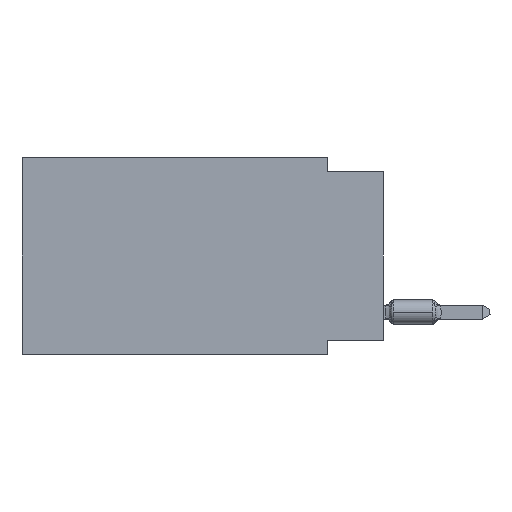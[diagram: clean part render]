
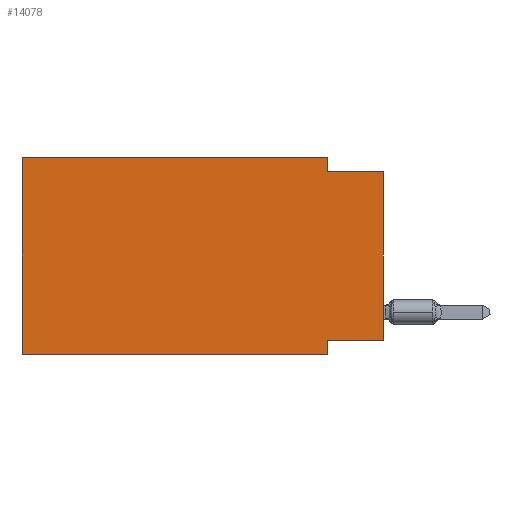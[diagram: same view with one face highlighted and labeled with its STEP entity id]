
A CAD part, left-side view. The second image highlights one B-rep face of the part: STEP entity #14078.
In plain terms, the highlighted planar face has unit normal (-1, 0, 0).
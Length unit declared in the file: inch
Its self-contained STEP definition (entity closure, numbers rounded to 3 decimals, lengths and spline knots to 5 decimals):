
#83 = VERTEX_POINT ( 'NONE', #13696 ) ;
#477 = EDGE_CURVE ( 'NONE', #13368, #14220, #11567, .T. ) ;
#613 = LINE ( 'NONE', #16002, #7493 ) ;
#871 = DIRECTION ( 'NONE',  ( 0., 0., 1. ) ) ;
#1409 = EDGE_CURVE ( 'NONE', #14233, #17961, #1791, .T. ) ;
#1791 = LINE ( 'NONE', #1878, #2820 ) ;
#1878 = CARTESIAN_POINT ( 'NONE',  ( 0., 0., -0.325 ) ) ;
#1926 = CARTESIAN_POINT ( 'NONE',  ( 0., 0.1, -0.025 ) ) ;
#2315 = VECTOR ( 'NONE', #11634, 39.37008 ) ;
#2380 = CARTESIAN_POINT ( 'NONE',  ( 0., 0.645, -0.35 ) ) ;
#2670 = FACE_OUTER_BOUND ( 'NONE', #18024, .T. ) ;
#2742 = ORIENTED_EDGE ( 'NONE', *, *, #7738, .F. ) ;
#2820 = VECTOR ( 'NONE', #7370, 39.37008 ) ;
#2941 = LINE ( 'NONE', #5693, #15136 ) ;
#3067 = VERTEX_POINT ( 'NONE', #17704 ) ;
#3193 = CARTESIAN_POINT ( 'NONE',  ( 0., 0., -0.325 ) ) ;
#3515 = AXIS2_PLACEMENT_3D ( 'NONE', #15423, #4151, #9726 ) ;
#3712 = CARTESIAN_POINT ( 'NONE',  ( 0., 0., -0.025 ) ) ;
#4151 = DIRECTION ( 'NONE',  ( 1., 0., 0. ) ) ;
#4336 = EDGE_CURVE ( 'NONE', #5197, #14372, #613, .T. ) ;
#4596 = ORIENTED_EDGE ( 'NONE', *, *, #477, .F. ) ;
#4948 = CARTESIAN_POINT ( 'NONE',  ( 0., 0.1, -0.35 ) ) ;
#5197 = VERTEX_POINT ( 'NONE', #2380 ) ;
#5522 = DIRECTION ( 'NONE',  ( 0., -1., 0. ) ) ;
#5693 = CARTESIAN_POINT ( 'NONE',  ( 0., 0.645, 0. ) ) ;
#6362 = DIRECTION ( 'NONE',  ( 0., -1., 0. ) ) ;
#6454 = DIRECTION ( 'NONE',  ( 0., -1., 0. ) ) ;
#7370 = DIRECTION ( 'NONE',  ( 0., 1., 0. ) ) ;
#7493 = VECTOR ( 'NONE', #6454, 39.37008 ) ;
#7738 = EDGE_CURVE ( 'NONE', #3067, #13368, #2941, .T. ) ;
#8234 = ORIENTED_EDGE ( 'NONE', *, *, #1409, .F. ) ;
#8845 = VECTOR ( 'NONE', #871, 39.37008 ) ;
#8878 = LINE ( 'NONE', #10259, #2315 ) ;
#9372 = EDGE_CURVE ( 'NONE', #17961, #14372, #15315, .T. ) ;
#9550 = ORIENTED_EDGE ( 'NONE', *, *, #12881, .F. ) ;
#9726 = DIRECTION ( 'NONE',  ( 0., 0., -1. ) ) ;
#9910 = EDGE_CURVE ( 'NONE', #14220, #83, #17641, .T. ) ;
#10259 = CARTESIAN_POINT ( 'NONE',  ( 0., 0.645, 0. ) ) ;
#10940 = CARTESIAN_POINT ( 'NONE',  ( 0., 0.1, -0.325 ) ) ;
#11521 = CARTESIAN_POINT ( 'NONE',  ( 0., 0., 0. ) ) ;
#11567 = LINE ( 'NONE', #12768, #13896 ) ;
#11634 = DIRECTION ( 'NONE',  ( 0., 0., 1. ) ) ;
#12768 = CARTESIAN_POINT ( 'NONE',  ( 0., 0.1, 0. ) ) ;
#12811 = CARTESIAN_POINT ( 'NONE',  ( 0., 0.1, 0. ) ) ;
#12871 = ORIENTED_EDGE ( 'NONE', *, *, #16096, .T. ) ;
#12881 = EDGE_CURVE ( 'NONE', #5197, #3067, #8878, .T. ) ;
#12896 = LINE ( 'NONE', #11521, #8845 ) ;
#13368 = VERTEX_POINT ( 'NONE', #12811 ) ;
#13696 = CARTESIAN_POINT ( 'NONE',  ( 0., 0., -0.025 ) ) ;
#13896 = VECTOR ( 'NONE', #15527, 39.37008 ) ;
#13968 = ORIENTED_EDGE ( 'NONE', *, *, #4336, .T. ) ;
#14078 = ADVANCED_FACE ( 'NONE', ( #2670 ), #16705, .F. ) ;
#14220 = VERTEX_POINT ( 'NONE', #1926 ) ;
#14233 = VERTEX_POINT ( 'NONE', #3193 ) ;
#14372 = VERTEX_POINT ( 'NONE', #4948 ) ;
#14596 = ORIENTED_EDGE ( 'NONE', *, *, #9372, .F. ) ;
#15133 = CARTESIAN_POINT ( 'NONE',  ( 0., 0.1, -0.35 ) ) ;
#15136 = VECTOR ( 'NONE', #5522, 39.37008 ) ;
#15187 = VECTOR ( 'NONE', #6362, 39.37008 ) ;
#15315 = LINE ( 'NONE', #15133, #17215 ) ;
#15423 = CARTESIAN_POINT ( 'NONE',  ( 0., 0.645, 0. ) ) ;
#15527 = DIRECTION ( 'NONE',  ( 0., 0., -1. ) ) ;
#15933 = ORIENTED_EDGE ( 'NONE', *, *, #9910, .F. ) ;
#16002 = CARTESIAN_POINT ( 'NONE',  ( 0., 0.645, -0.35 ) ) ;
#16096 = EDGE_CURVE ( 'NONE', #14233, #83, #12896, .T. ) ;
#16688 = DIRECTION ( 'NONE',  ( 0., 0., -1. ) ) ;
#16705 = PLANE ( 'NONE',  #3515 ) ;
#17215 = VECTOR ( 'NONE', #16688, 39.37008 ) ;
#17641 = LINE ( 'NONE', #3712, #15187 ) ;
#17704 = CARTESIAN_POINT ( 'NONE',  ( 0., 0.645, 0. ) ) ;
#17961 = VERTEX_POINT ( 'NONE', #10940 ) ;
#18024 = EDGE_LOOP ( 'NONE', ( #12871, #15933, #4596, #2742, #9550, #13968, #14596, #8234 ) ) ;
